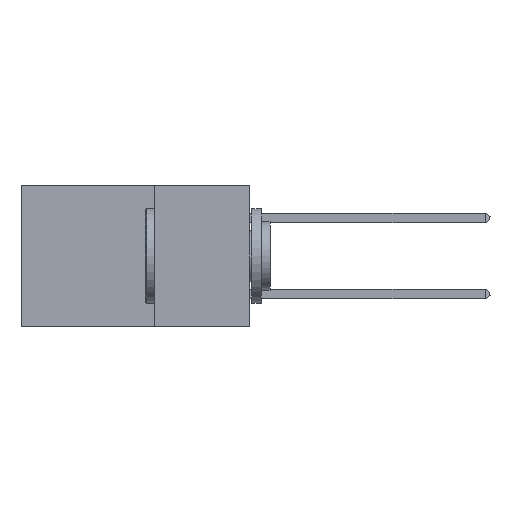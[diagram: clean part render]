
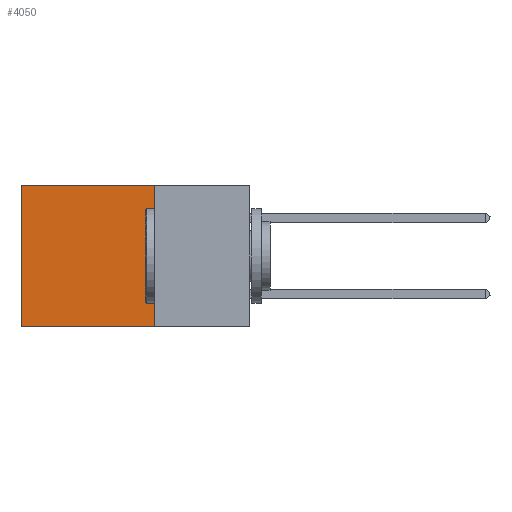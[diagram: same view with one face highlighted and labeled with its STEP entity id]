
A CAD part, left-side view. The second image highlights one B-rep face of the part: STEP entity #4050.
In plain terms, the highlighted planar face has unit normal (-1, 0, 0).
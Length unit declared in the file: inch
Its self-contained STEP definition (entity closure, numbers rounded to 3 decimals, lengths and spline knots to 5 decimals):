
#926 = CARTESIAN_POINT ( 'NONE',  ( 0.2875, 0.25, 0. ) ) ;
#2191 = DIRECTION ( 'NONE',  ( 0., 1., 0. ) ) ;
#3105 = DIRECTION ( 'NONE',  ( 0., 1., 0. ) ) ;
#3814 = CARTESIAN_POINT ( 'NONE',  ( 0.2875, 0.6, 0. ) ) ;
#4050 = ADVANCED_FACE ( 'NONE', ( #6388 ), #17750, .F. ) ;
#5511 = ORIENTED_EDGE ( 'NONE', *, *, #17435, .T. ) ;
#6238 = LINE ( 'NONE', #27207, #21174 ) ;
#6310 = CARTESIAN_POINT ( 'NONE',  ( 0.2875, 0.6, 0. ) ) ;
#6388 = FACE_OUTER_BOUND ( 'NONE', #29139, .T. ) ;
#7222 = ORIENTED_EDGE ( 'NONE', *, *, #25103, .T. ) ;
#7768 = EDGE_CURVE ( 'NONE', #32456, #14269, #6238, .T. ) ;
#8479 = CARTESIAN_POINT ( 'NONE',  ( 0.2875, 0.25, 0. ) ) ;
#9830 = DIRECTION ( 'NONE',  ( 0., 0., -1. ) ) ;
#10578 = ORIENTED_EDGE ( 'NONE', *, *, #7768, .F. ) ;
#12322 = DIRECTION ( 'NONE',  ( 1., 0., 0. ) ) ;
#12507 = VERTEX_POINT ( 'NONE', #21975 ) ;
#12525 = EDGE_CURVE ( 'NONE', #14269, #12507, #36572, .T. ) ;
#13576 = AXIS2_PLACEMENT_3D ( 'NONE', #26565, #12322, #32622 ) ;
#14024 = LINE ( 'NONE', #3814, #25841 ) ;
#14269 = VERTEX_POINT ( 'NONE', #35839 ) ;
#17435 = EDGE_CURVE ( 'NONE', #31685, #12507, #14024, .T. ) ;
#17750 = PLANE ( 'NONE',  #13576 ) ;
#18674 = ORIENTED_EDGE ( 'NONE', *, *, #12525, .F. ) ;
#21174 = VECTOR ( 'NONE', #9830, 39.37008 ) ;
#21975 = CARTESIAN_POINT ( 'NONE',  ( 0.2875, 0.6, -0.37 ) ) ;
#25103 = EDGE_CURVE ( 'NONE', #32456, #31685, #35478, .T. ) ;
#25841 = VECTOR ( 'NONE', #29986, 39.37008 ) ;
#26565 = CARTESIAN_POINT ( 'NONE',  ( 0.2875, 0.25, 0. ) ) ;
#27207 = CARTESIAN_POINT ( 'NONE',  ( 0.2875, 0.25, 0. ) ) ;
#27578 = VECTOR ( 'NONE', #2191, 39.37008 ) ;
#27820 = VECTOR ( 'NONE', #3105, 39.37008 ) ;
#29139 = EDGE_LOOP ( 'NONE', ( #5511, #18674, #10578, #7222 ) ) ;
#29986 = DIRECTION ( 'NONE',  ( 0., 0., -1. ) ) ;
#31685 = VERTEX_POINT ( 'NONE', #6310 ) ;
#32456 = VERTEX_POINT ( 'NONE', #926 ) ;
#32622 = DIRECTION ( 'NONE',  ( 0., 0., -1. ) ) ;
#34036 = CARTESIAN_POINT ( 'NONE',  ( 0.2875, 0.25, -0.37 ) ) ;
#35478 = LINE ( 'NONE', #8479, #27820 ) ;
#35839 = CARTESIAN_POINT ( 'NONE',  ( 0.2875, 0.25, -0.37 ) ) ;
#36572 = LINE ( 'NONE', #34036, #27578 ) ;
